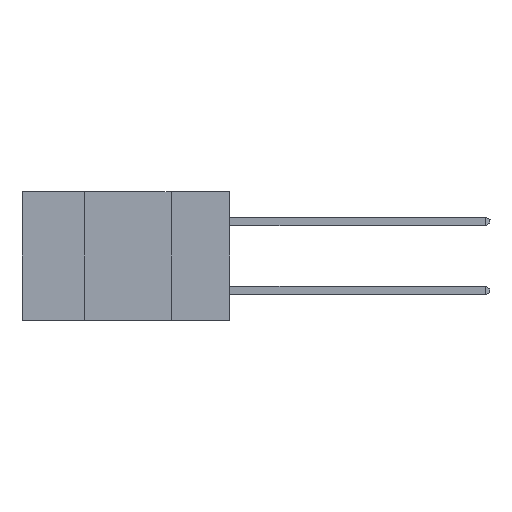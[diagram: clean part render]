
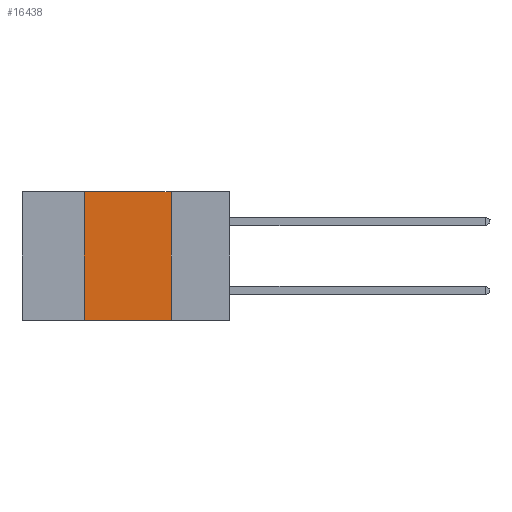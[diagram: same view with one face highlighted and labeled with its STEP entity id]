
A CAD part, left-side view. The second image highlights one B-rep face of the part: STEP entity #16438.
In plain terms, the highlighted planar face has unit normal (-1, 0, 0).
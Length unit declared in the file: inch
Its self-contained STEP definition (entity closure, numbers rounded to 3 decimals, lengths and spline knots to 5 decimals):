
#215 = VECTOR ( 'NONE', #5842, 39.37008 ) ;
#567 = DIRECTION ( 'NONE',  ( 0., 0., 1. ) ) ;
#1407 = VERTEX_POINT ( 'NONE', #6951 ) ;
#1792 = PLANE ( 'NONE',  #14378 ) ;
#1842 = DIRECTION ( 'NONE',  ( 0., 0., -1. ) ) ;
#2432 = VECTOR ( 'NONE', #1842, 39.37008 ) ;
#3287 = ORIENTED_EDGE ( 'NONE', *, *, #8336, .F. ) ;
#3362 = ORIENTED_EDGE ( 'NONE', *, *, #4363, .T. ) ;
#4187 = ORIENTED_EDGE ( 'NONE', *, *, #12398, .F. ) ;
#4363 = EDGE_CURVE ( 'NONE', #1407, #6746, #13156, .T. ) ;
#4469 = CARTESIAN_POINT ( 'NONE',  ( 0., 0.42, 0. ) ) ;
#4511 = CARTESIAN_POINT ( 'NONE',  ( 0., 0.6, 0. ) ) ;
#5468 = EDGE_CURVE ( 'NONE', #9942, #6746, #6350, .T. ) ;
#5842 = DIRECTION ( 'NONE',  ( 0., -1., 0. ) ) ;
#6227 = LINE ( 'NONE', #7796, #14224 ) ;
#6350 = LINE ( 'NONE', #14953, #2432 ) ;
#6746 = VERTEX_POINT ( 'NONE', #12535 ) ;
#6951 = CARTESIAN_POINT ( 'NONE',  ( 0., 0.42, -0.37 ) ) ;
#7796 = CARTESIAN_POINT ( 'NONE',  ( 0., 0.6, 0. ) ) ;
#7859 = DIRECTION ( 'NONE',  ( 0., -1., 0. ) ) ;
#8261 = CARTESIAN_POINT ( 'NONE',  ( 0., 0.17, 0. ) ) ;
#8336 = EDGE_CURVE ( 'NONE', #1407, #14641, #9740, .T. ) ;
#8454 = CARTESIAN_POINT ( 'NONE',  ( 0., 0.42, 0. ) ) ;
#8823 = EDGE_LOOP ( 'NONE', ( #11723, #4187, #3287, #3362 ) ) ;
#8926 = VECTOR ( 'NONE', #567, 39.37008 ) ;
#9740 = LINE ( 'NONE', #8454, #8926 ) ;
#9942 = VERTEX_POINT ( 'NONE', #8261 ) ;
#11723 = ORIENTED_EDGE ( 'NONE', *, *, #5468, .F. ) ;
#12304 = DIRECTION ( 'NONE',  ( 1., 0., 0. ) ) ;
#12398 = EDGE_CURVE ( 'NONE', #14641, #9942, #6227, .T. ) ;
#12535 = CARTESIAN_POINT ( 'NONE',  ( 0., 0.17, -0.37 ) ) ;
#13156 = LINE ( 'NONE', #16110, #215 ) ;
#14224 = VECTOR ( 'NONE', #7859, 39.37008 ) ;
#14378 = AXIS2_PLACEMENT_3D ( 'NONE', #4511, #12304, #15088 ) ;
#14641 = VERTEX_POINT ( 'NONE', #4469 ) ;
#14953 = CARTESIAN_POINT ( 'NONE',  ( 0., 0.17, 0. ) ) ;
#15088 = DIRECTION ( 'NONE',  ( 0., 0., -1. ) ) ;
#16110 = CARTESIAN_POINT ( 'NONE',  ( 0., 0.6, -0.37 ) ) ;
#16339 = FACE_OUTER_BOUND ( 'NONE', #8823, .T. ) ;
#16438 = ADVANCED_FACE ( 'NONE', ( #16339 ), #1792, .F. ) ;
